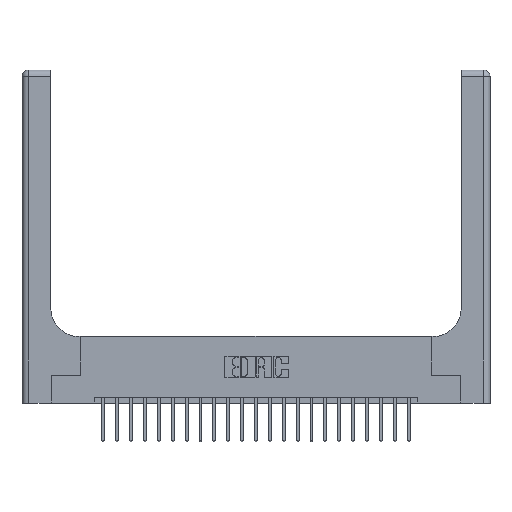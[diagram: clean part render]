
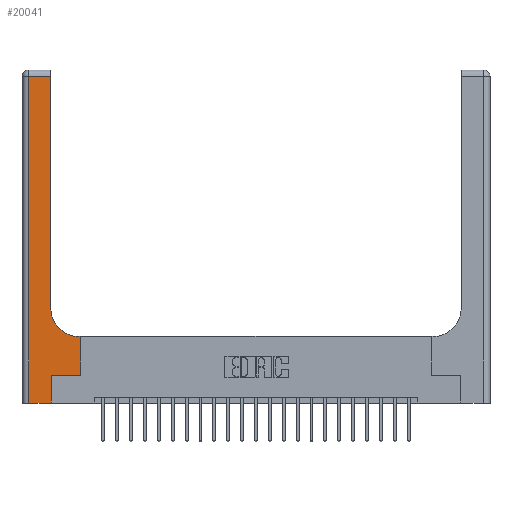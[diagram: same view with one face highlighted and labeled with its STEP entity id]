
A CAD part, top view. The second image highlights one B-rep face of the part: STEP entity #20041.
In plain terms, the highlighted planar face has unit normal (0, 0, 1).
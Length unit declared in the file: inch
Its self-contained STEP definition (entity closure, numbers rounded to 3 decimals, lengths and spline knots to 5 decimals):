
#728 = VERTEX_POINT ( 'NONE', #19157 ) ;
#899 = DIRECTION ( 'NONE',  ( 0., 1., 0. ) ) ;
#1209 = LINE ( 'NONE', #11372, #5320 ) ;
#1503 = DIRECTION ( 'NONE',  ( -1., 0., 0. ) ) ;
#1690 = EDGE_CURVE ( 'NONE', #11592, #18737, #18502, .T. ) ;
#2167 = ORIENTED_EDGE ( 'NONE', *, *, #17721, .T. ) ;
#2222 = VERTEX_POINT ( 'NONE', #18155 ) ;
#2329 = DIRECTION ( 'NONE',  ( 0., 1., 0. ) ) ;
#2684 = EDGE_CURVE ( 'NONE', #2222, #728, #14627, .T. ) ;
#3180 = AXIS2_PLACEMENT_3D ( 'NONE', #9216, #3982, #3910 ) ;
#3498 = CARTESIAN_POINT ( 'NONE',  ( 0., 2.94, 0.37 ) ) ;
#3593 = CARTESIAN_POINT ( 'NONE',  ( 0.265, 0.25, 0.37 ) ) ;
#3655 = DIRECTION ( 'NONE',  ( 1., 0., 0. ) ) ;
#3910 = DIRECTION ( 'NONE',  ( -1., 0., 0. ) ) ;
#3982 = DIRECTION ( 'NONE',  ( 0., 0., -1. ) ) ;
#4214 = PLANE ( 'NONE',  #3180 ) ;
#4421 = EDGE_CURVE ( 'NONE', #11336, #9820, #16744, .T. ) ;
#5320 = VECTOR ( 'NONE', #11522, 39.37008 ) ;
#5396 = VECTOR ( 'NONE', #899, 39.37008 ) ;
#5511 = CARTESIAN_POINT ( 'NONE',  ( 0.51, 0.6, 0.37 ) ) ;
#5957 = EDGE_CURVE ( 'NONE', #16418, #17796, #14705, .T. ) ;
#6116 = ORIENTED_EDGE ( 'NONE', *, *, #17584, .T. ) ;
#7185 = CARTESIAN_POINT ( 'NONE',  ( 0.51, 0.85, 0.37 ) ) ;
#7285 = DIRECTION ( 'NONE',  ( 0., 1., 0. ) ) ;
#7455 = CARTESIAN_POINT ( 'NONE',  ( 0.528, 0.25, 0.37 ) ) ;
#7721 = ORIENTED_EDGE ( 'NONE', *, *, #9686, .T. ) ;
#8269 = CARTESIAN_POINT ( 'NONE',  ( 0.26, 0.6, 0.37 ) ) ;
#8388 = EDGE_LOOP ( 'NONE', ( #9290, #12424, #6116, #7721, #22559, #19883, #17527, #2167, #10650 ) ) ;
#9216 = CARTESIAN_POINT ( 'NONE',  ( 0., 3., 0.37 ) ) ;
#9290 = ORIENTED_EDGE ( 'NONE', *, *, #20202, .T. ) ;
#9686 = EDGE_CURVE ( 'NONE', #21731, #16418, #18455, .T. ) ;
#9820 = VERTEX_POINT ( 'NONE', #17860 ) ;
#10279 = CARTESIAN_POINT ( 'NONE',  ( 0.06, 0., 0.37 ) ) ;
#10650 = ORIENTED_EDGE ( 'NONE', *, *, #4421, .T. ) ;
#10770 = CARTESIAN_POINT ( 'NONE',  ( 0.265, 0., 0.37 ) ) ;
#11218 = AXIS2_PLACEMENT_3D ( 'NONE', #7185, #19513, #19201 ) ;
#11336 = VERTEX_POINT ( 'NONE', #5511 ) ;
#11372 = CARTESIAN_POINT ( 'NONE',  ( 0.06, 3., 0.37 ) ) ;
#11488 = FACE_OUTER_BOUND ( 'NONE', #8388, .T. ) ;
#11503 = CARTESIAN_POINT ( 'NONE',  ( 0.26, 3., 0.37 ) ) ;
#11522 = DIRECTION ( 'NONE',  ( 0., -1., 0. ) ) ;
#11550 = CARTESIAN_POINT ( 'NONE',  ( 0.528, 0.6, 0.37 ) ) ;
#11592 = VERTEX_POINT ( 'NONE', #20142 ) ;
#11595 = VECTOR ( 'NONE', #1503, 39.37008 ) ;
#11669 = VECTOR ( 'NONE', #7285, 39.37008 ) ;
#12009 = LINE ( 'NONE', #11503, #5396 ) ;
#12120 = VECTOR ( 'NONE', #3655, 39.37008 ) ;
#12424 = ORIENTED_EDGE ( 'NONE', *, *, #2684, .T. ) ;
#12639 = EDGE_CURVE ( 'NONE', #17796, #11592, #13257, .T. ) ;
#12843 = DIRECTION ( 'NONE',  ( 1., 0., 0. ) ) ;
#13257 = LINE ( 'NONE', #14204, #12120 ) ;
#13552 = VECTOR ( 'NONE', #12843, 39.37008 ) ;
#14204 = CARTESIAN_POINT ( 'NONE',  ( 0.265, 0.25, 0.37 ) ) ;
#14464 = CARTESIAN_POINT ( 'NONE',  ( 0., 0., 0.37 ) ) ;
#14627 = LINE ( 'NONE', #3498, #11595 ) ;
#14705 = LINE ( 'NONE', #10770, #11669 ) ;
#15346 = CARTESIAN_POINT ( 'NONE',  ( 0.265, 0., 0.37 ) ) ;
#16418 = VERTEX_POINT ( 'NONE', #15346 ) ;
#16608 = VECTOR ( 'NONE', #2329, 39.37008 ) ;
#16744 = CIRCLE ( 'NONE', #11218, 0.25 ) ;
#17527 = ORIENTED_EDGE ( 'NONE', *, *, #1690, .T. ) ;
#17584 = EDGE_CURVE ( 'NONE', #728, #21731, #1209, .T. ) ;
#17721 = EDGE_CURVE ( 'NONE', #18737, #11336, #21303, .T. ) ;
#17796 = VERTEX_POINT ( 'NONE', #3593 ) ;
#17860 = CARTESIAN_POINT ( 'NONE',  ( 0.26, 0.85, 0.37 ) ) ;
#18155 = CARTESIAN_POINT ( 'NONE',  ( 0.26, 2.94, 0.37 ) ) ;
#18455 = LINE ( 'NONE', #14464, #13552 ) ;
#18502 = LINE ( 'NONE', #7455, #16608 ) ;
#18737 = VERTEX_POINT ( 'NONE', #11550 ) ;
#18954 = DIRECTION ( 'NONE',  ( -1., 0., 0. ) ) ;
#19157 = CARTESIAN_POINT ( 'NONE',  ( 0.06, 2.94, 0.37 ) ) ;
#19201 = DIRECTION ( 'NONE',  ( 1., 0., 0. ) ) ;
#19513 = DIRECTION ( 'NONE',  ( 0., 0., -1. ) ) ;
#19883 = ORIENTED_EDGE ( 'NONE', *, *, #12639, .T. ) ;
#19915 = VECTOR ( 'NONE', #18954, 39.37008 ) ;
#20041 = ADVANCED_FACE ( 'NONE', ( #11488 ), #4214, .F. ) ;
#20142 = CARTESIAN_POINT ( 'NONE',  ( 0.528, 0.25, 0.37 ) ) ;
#20202 = EDGE_CURVE ( 'NONE', #9820, #2222, #12009, .T. ) ;
#21303 = LINE ( 'NONE', #8269, #19915 ) ;
#21731 = VERTEX_POINT ( 'NONE', #10279 ) ;
#22559 = ORIENTED_EDGE ( 'NONE', *, *, #5957, .T. ) ;
